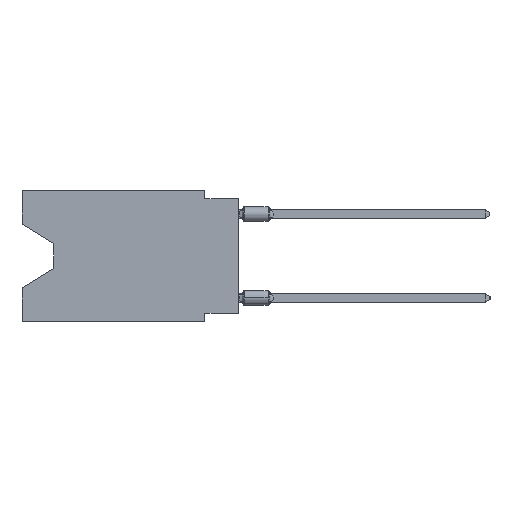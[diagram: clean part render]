
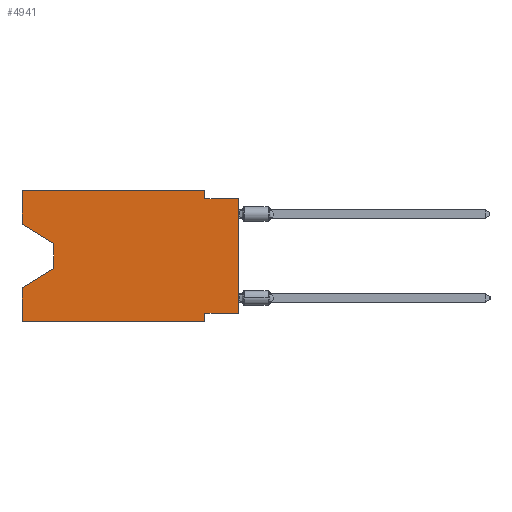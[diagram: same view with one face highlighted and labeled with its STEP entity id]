
A CAD part, left-side view. The second image highlights one B-rep face of the part: STEP entity #4941.
In plain terms, the highlighted planar face has unit normal (-1, 0, 0).
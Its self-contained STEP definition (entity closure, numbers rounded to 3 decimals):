
#400 = VECTOR ( 'NONE', #21592, 1000. ) ;
#510 = CARTESIAN_POINT ( 'NONE',  ( 0., 0., -9.271 ) ) ;
#1105 = ORIENTED_EDGE ( 'NONE', *, *, #13660, .F. ) ;
#1524 = VERTEX_POINT ( 'NONE', #2046 ) ;
#1901 = EDGE_CURVE ( 'NONE', #43738, #58982, #30413, .T. ) ;
#1902 = LINE ( 'NONE', #37046, #29003 ) ;
#2046 = CARTESIAN_POINT ( 'NONE',  ( 0., 0., -9.271 ) ) ;
#2834 = ORIENTED_EDGE ( 'NONE', *, *, #40550, .F. ) ;
#2836 = EDGE_CURVE ( 'NONE', #44062, #18426, #17588, .T. ) ;
#3583 = EDGE_CURVE ( 'NONE', #47251, #5253, #39339, .T. ) ;
#4686 = CARTESIAN_POINT ( 'NONE',  ( 0., 16.383, 0. ) ) ;
#4941 = ADVANCED_FACE ( 'NONE', ( #12663 ), #54017, .F. ) ;
#4991 = DIRECTION ( 'NONE',  ( 0., -1., 0. ) ) ;
#5253 = VERTEX_POINT ( 'NONE', #59001 ) ;
#5359 = CARTESIAN_POINT ( 'NONE',  ( 0., 16.383, 0. ) ) ;
#6663 = CARTESIAN_POINT ( 'NONE',  ( 0., 16.383, -2.546 ) ) ;
#6930 = VECTOR ( 'NONE', #39707, 1000. ) ;
#7048 = CARTESIAN_POINT ( 'NONE',  ( 0., 16.383, -9.906 ) ) ;
#7463 = ORIENTED_EDGE ( 'NONE', *, *, #11031, .F. ) ;
#7588 = VERTEX_POINT ( 'NONE', #50495 ) ;
#8308 = LINE ( 'NONE', #35289, #50559 ) ;
#8339 = VERTEX_POINT ( 'NONE', #50359 ) ;
#8631 = ORIENTED_EDGE ( 'NONE', *, *, #28013, .F. ) ;
#8776 = CARTESIAN_POINT ( 'NONE',  ( 0., 0., -0.635 ) ) ;
#9179 = CARTESIAN_POINT ( 'NONE',  ( 0., 16.383, 0. ) ) ;
#10702 = VECTOR ( 'NONE', #12871, 1000. ) ;
#10768 = EDGE_CURVE ( 'NONE', #8339, #7588, #26347, .T. ) ;
#11031 = EDGE_CURVE ( 'NONE', #47251, #44062, #19722, .T. ) ;
#11612 = VECTOR ( 'NONE', #4991, 1000. ) ;
#12663 = FACE_OUTER_BOUND ( 'NONE', #30839, .T. ) ;
#12871 = DIRECTION ( 'NONE',  ( 0., 0.855, -0.519 ) ) ;
#13251 = ORIENTED_EDGE ( 'NONE', *, *, #3583, .T. ) ;
#13660 = EDGE_CURVE ( 'NONE', #18426, #22879, #16487, .T. ) ;
#13769 = LINE ( 'NONE', #35675, #52086 ) ;
#13877 = EDGE_CURVE ( 'NONE', #1524, #45798, #13769, .T. ) ;
#13954 = LINE ( 'NONE', #4686, #48533 ) ;
#14393 = VECTOR ( 'NONE', #55945, 1000. ) ;
#16487 = LINE ( 'NONE', #29995, #400 ) ;
#17068 = CARTESIAN_POINT ( 'NONE',  ( 0., 13.97, -5.893 ) ) ;
#17378 = DIRECTION ( 'NONE',  ( 0., 0., 1. ) ) ;
#17588 = LINE ( 'NONE', #9179, #11612 ) ;
#18341 = DIRECTION ( 'NONE',  ( 1., 0., 0. ) ) ;
#18423 = ORIENTED_EDGE ( 'NONE', *, *, #2836, .F. ) ;
#18426 = VERTEX_POINT ( 'NONE', #55839 ) ;
#18466 = DIRECTION ( 'NONE',  ( 0., 0., -1. ) ) ;
#18974 = EDGE_CURVE ( 'NONE', #44094, #58982, #8308, .T. ) ;
#19722 = LINE ( 'NONE', #5359, #33677 ) ;
#20317 = VECTOR ( 'NONE', #56737, 1000. ) ;
#21592 = DIRECTION ( 'NONE',  ( 0., 0., -1. ) ) ;
#21960 = CARTESIAN_POINT ( 'NONE',  ( 0., 16.383, 0. ) ) ;
#22879 = VERTEX_POINT ( 'NONE', #48484 ) ;
#24992 = CARTESIAN_POINT ( 'NONE',  ( 0., 2.54, -9.906 ) ) ;
#26347 = LINE ( 'NONE', #17068, #10702 ) ;
#26935 = CARTESIAN_POINT ( 'NONE',  ( 0., 2.54, -9.271 ) ) ;
#28013 = EDGE_CURVE ( 'NONE', #43738, #7588, #13954, .T. ) ;
#29003 = VECTOR ( 'NONE', #18466, 1000. ) ;
#29995 = CARTESIAN_POINT ( 'NONE',  ( 0., 2.54, 0. ) ) ;
#30254 = EDGE_CURVE ( 'NONE', #1524, #44094, #32878, .T. ) ;
#30413 = LINE ( 'NONE', #7048, #6930 ) ;
#30839 = EDGE_LOOP ( 'NONE', ( #13251, #41343, #52695, #8631, #37739, #38186, #31246, #49195, #2834, #1105, #18423, #7463 ) ) ;
#31246 = ORIENTED_EDGE ( 'NONE', *, *, #30254, .F. ) ;
#31255 = DIRECTION ( 'NONE',  ( 0., 0., -1. ) ) ;
#32878 = LINE ( 'NONE', #510, #14393 ) ;
#33677 = VECTOR ( 'NONE', #52387, 1000. ) ;
#33718 = EDGE_CURVE ( 'NONE', #5253, #8339, #1902, .T. ) ;
#35289 = CARTESIAN_POINT ( 'NONE',  ( 0., 2.54, -9.906 ) ) ;
#35675 = CARTESIAN_POINT ( 'NONE',  ( 0., 0., 0. ) ) ;
#36650 = LINE ( 'NONE', #8776, #58268 ) ;
#37046 = CARTESIAN_POINT ( 'NONE',  ( 0., 13.97, -4.013 ) ) ;
#37739 = ORIENTED_EDGE ( 'NONE', *, *, #1901, .T. ) ;
#38186 = ORIENTED_EDGE ( 'NONE', *, *, #18974, .F. ) ;
#39339 = LINE ( 'NONE', #52532, #20317 ) ;
#39707 = DIRECTION ( 'NONE',  ( 0., -1., 0. ) ) ;
#40438 = CARTESIAN_POINT ( 'NONE',  ( 0., 16.383, 0. ) ) ;
#40550 = EDGE_CURVE ( 'NONE', #22879, #45798, #36650, .T. ) ;
#41343 = ORIENTED_EDGE ( 'NONE', *, *, #33718, .T. ) ;
#43429 = AXIS2_PLACEMENT_3D ( 'NONE', #21960, #18341, #31255 ) ;
#43738 = VERTEX_POINT ( 'NONE', #56650 ) ;
#44062 = VERTEX_POINT ( 'NONE', #40438 ) ;
#44094 = VERTEX_POINT ( 'NONE', #26935 ) ;
#45798 = VERTEX_POINT ( 'NONE', #54033 ) ;
#45946 = DIRECTION ( 'NONE',  ( 0., -1., 0. ) ) ;
#47251 = VERTEX_POINT ( 'NONE', #6663 ) ;
#48484 = CARTESIAN_POINT ( 'NONE',  ( 0., 2.54, -0.635 ) ) ;
#48533 = VECTOR ( 'NONE', #54431, 1000. ) ;
#49195 = ORIENTED_EDGE ( 'NONE', *, *, #13877, .T. ) ;
#50359 = CARTESIAN_POINT ( 'NONE',  ( 0., 13.97, -5.893 ) ) ;
#50495 = CARTESIAN_POINT ( 'NONE',  ( 0., 16.383, -7.36 ) ) ;
#50559 = VECTOR ( 'NONE', #58942, 1000. ) ;
#52086 = VECTOR ( 'NONE', #17378, 1000. ) ;
#52387 = DIRECTION ( 'NONE',  ( 0., 0., 1. ) ) ;
#52532 = CARTESIAN_POINT ( 'NONE',  ( 0., 16.383, -2.546 ) ) ;
#52695 = ORIENTED_EDGE ( 'NONE', *, *, #10768, .T. ) ;
#54017 = PLANE ( 'NONE',  #43429 ) ;
#54033 = CARTESIAN_POINT ( 'NONE',  ( 0., 0., -0.635 ) ) ;
#54431 = DIRECTION ( 'NONE',  ( 0., 0., 1. ) ) ;
#55839 = CARTESIAN_POINT ( 'NONE',  ( 0., 2.54, 0. ) ) ;
#55945 = DIRECTION ( 'NONE',  ( 0., 1., 0. ) ) ;
#56650 = CARTESIAN_POINT ( 'NONE',  ( 0., 16.383, -9.906 ) ) ;
#56737 = DIRECTION ( 'NONE',  ( 0., -0.855, -0.519 ) ) ;
#58268 = VECTOR ( 'NONE', #45946, 1000. ) ;
#58942 = DIRECTION ( 'NONE',  ( 0., 0., -1. ) ) ;
#58982 = VERTEX_POINT ( 'NONE', #24992 ) ;
#59001 = CARTESIAN_POINT ( 'NONE',  ( 0., 13.97, -4.013 ) ) ;
